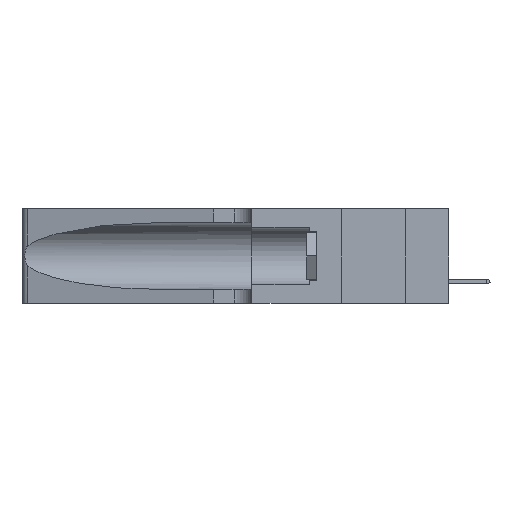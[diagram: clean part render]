
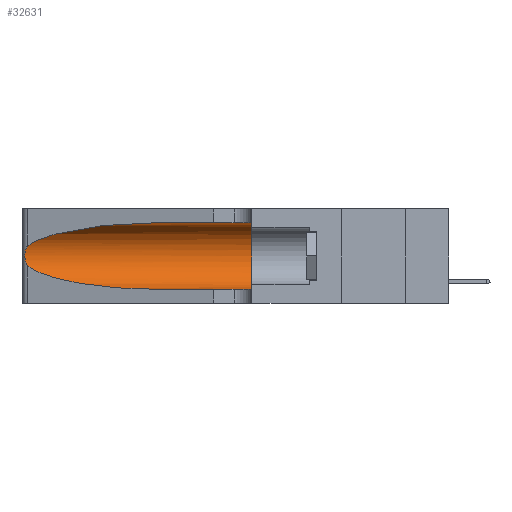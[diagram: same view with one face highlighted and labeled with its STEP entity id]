
A CAD part, left-side view. The second image highlights one B-rep face of the part: STEP entity #32631.
In plain terms, the highlighted cylindrical face has radius 3.308 mm (diameter 6.617 mm), a partial arc.
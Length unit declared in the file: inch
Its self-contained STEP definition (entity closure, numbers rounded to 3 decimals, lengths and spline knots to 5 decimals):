
#422 = CARTESIAN_POINT ( 'NONE',  ( 0.26017, 1.23833, 0.17102 ) ) ;
#545 = EDGE_CURVE ( 'NONE', #37888, #43125, #31810, .T. ) ;
#982 = VERTEX_POINT ( 'NONE', #29966 ) ;
#1101 = CARTESIAN_POINT ( 'NONE',  ( 0.1305, 1.61858, 0.05475 ) ) ;
#1634 = VERTEX_POINT ( 'NONE', #4740 ) ;
#1874 = DIRECTION ( 'NONE',  ( 0., -1., 0. ) ) ;
#2997 = VERTEX_POINT ( 'NONE', #22173 ) ;
#4637 = CARTESIAN_POINT ( 'NONE',  ( 0.25487, 1.22718, 0.22369 ) ) ;
#4740 = CARTESIAN_POINT ( 'NONE',  ( 0.1305, 0.72297, 0.31525 ) ) ;
#6205 = AXIS2_PLACEMENT_3D ( 'NONE', #44078, #36789, #33046 ) ;
#6620 = FACE_OUTER_BOUND ( 'NONE', #32983, .T. ) ;
#6722 = ORIENTED_EDGE ( 'NONE', *, *, #46724, .T. ) ;
#7858 = CARTESIAN_POINT ( 'NONE',  ( 0.25789, 1.23486, 0.15765 ) ) ;
#9179 = CARTESIAN_POINT ( 'NONE',  ( 0.1305, 1.61858, 0.185 ) ) ;
#10398 = EDGE_CURVE ( 'NONE', #982, #2997, #11980, .T. ) ;
#11980 =( BOUNDED_CURVE ( )  B_SPLINE_CURVE ( 3, ( #13541, #35560, #21111, #28175 ),
 .UNSPECIFIED., .F., .F. ) 
 B_SPLINE_CURVE_WITH_KNOTS ( ( 4, 4 ),
 ( 3.44316, 4.71239 ),
 .UNSPECIFIED. ) 
 CURVE ( )  GEOMETRIC_REPRESENTATION_ITEM ( )  RATIONAL_B_SPLINE_CURVE ( ( 1., 0.87, 0.87, 1. ) ) 
 REPRESENTATION_ITEM ( '' )  );
#12842 = ORIENTED_EDGE ( 'NONE', *, *, #17609, .F. ) ;
#13142 = VERTEX_POINT ( 'NONE', #40072 ) ;
#13541 = CARTESIAN_POINT ( 'NONE',  ( 0.25487, 1.22718, 0.14631 ) ) ;
#13623 = ORIENTED_EDGE ( 'NONE', *, *, #23162, .T. ) ;
#14616 = LINE ( 'NONE', #41097, #32411 ) ;
#14864 = LINE ( 'NONE', #1101, #34340 ) ;
#15486 = CARTESIAN_POINT ( 'NONE',  ( 0.25856, 1.23593, 0.16098 ) ) ;
#17253 = AXIS2_PLACEMENT_3D ( 'NONE', #9179, #1874, #26870 ) ;
#17609 = EDGE_CURVE ( 'NONE', #1634, #37888, #14616, .T. ) ;
#18834 = CARTESIAN_POINT ( 'NONE',  ( 0.25555, 1.22993, 0.14849 ) ) ;
#19293 = CARTESIAN_POINT ( 'NONE',  ( 0.2373, 1.15595, 0.28018 ) ) ;
#19314 = CARTESIAN_POINT ( 'NONE',  ( 0.25639, 1.23184, 0.21858 ) ) ;
#19523 = DIRECTION ( 'NONE',  ( 0., -1., 0. ) ) ;
#19613 = CARTESIAN_POINT ( 'NONE',  ( 0.25487, 1.22718, 0.22369 ) ) ;
#20536 = B_SPLINE_CURVE_WITH_KNOTS ( 'NONE', 3,
 ( #4637, #40883, #19314, #30247, #33598, #33901, #44627, #26228, #422, #15486, #7858, #22690, #18834, #41204 ),
 .UNSPECIFIED., .F., .F.,
 ( 4, 2, 2, 2, 2, 2, 4 ),
 ( 0., 0.00027, 0.00053, 0.00107, 0.0016, 0.00187, 0.00214 ),
 .UNSPECIFIED. ) ;
#20895 = EDGE_CURVE ( 'NONE', #2997, #43125, #14864, .T. ) ;
#21111 = CARTESIAN_POINT ( 'NONE',  ( 0.18966, 0.96281, 0.05475 ) ) ;
#21895 = CARTESIAN_POINT ( 'NONE',  ( 0.1305, 0.35, 0.31525 ) ) ;
#22173 = CARTESIAN_POINT ( 'NONE',  ( 0.1305, 0.72297, 0.05475 ) ) ;
#22690 = CARTESIAN_POINT ( 'NONE',  ( 0.25639, 1.23186, 0.15144 ) ) ;
#22770 = ORIENTED_EDGE ( 'NONE', *, *, #545, .F. ) ;
#23162 = EDGE_CURVE ( 'NONE', #1634, #13142, #36978, .T. ) ;
#23308 = CARTESIAN_POINT ( 'NONE',  ( 0.18966, 0.96281, 0.31525 ) ) ;
#23467 = CARTESIAN_POINT ( 'NONE',  ( 0.1305, 0.72297, 0.31525 ) ) ;
#24343 = CYLINDRICAL_SURFACE ( 'NONE', #17253, 0.13025 ) ;
#26228 = CARTESIAN_POINT ( 'NONE',  ( 0.26075, 1.23896, 0.178 ) ) ;
#26870 = DIRECTION ( 'NONE',  ( 0., 0., -1. ) ) ;
#28175 = CARTESIAN_POINT ( 'NONE',  ( 0.1305, 0.72297, 0.05475 ) ) ;
#29966 = CARTESIAN_POINT ( 'NONE',  ( 0.25487, 1.22718, 0.14631 ) ) ;
#30247 = CARTESIAN_POINT ( 'NONE',  ( 0.25787, 1.23484, 0.2124 ) ) ;
#31810 = CIRCLE ( 'NONE', #6205, 0.13025 ) ;
#32411 = VECTOR ( 'NONE', #19523, 39.37008 ) ;
#32631 = ADVANCED_FACE ( 'NONE', ( #6620 ), #24343, .F. ) ;
#32983 = EDGE_LOOP ( 'NONE', ( #13623, #6722, #38938, #36609, #22770, #12842 ) ) ;
#33046 = DIRECTION ( 'NONE',  ( 0., 0., 1. ) ) ;
#33598 = CARTESIAN_POINT ( 'NONE',  ( 0.25854, 1.2359, 0.20912 ) ) ;
#33901 = CARTESIAN_POINT ( 'NONE',  ( 0.26018, 1.23835, 0.19895 ) ) ;
#34340 = VECTOR ( 'NONE', #42458, 39.37008 ) ;
#35560 = CARTESIAN_POINT ( 'NONE',  ( 0.2373, 1.15595, 0.08982 ) ) ;
#36609 = ORIENTED_EDGE ( 'NONE', *, *, #20895, .T. ) ;
#36789 = DIRECTION ( 'NONE',  ( 0., 1., 0. ) ) ;
#36978 =( BOUNDED_CURVE ( )  B_SPLINE_CURVE ( 3, ( #23467, #23308, #19293, #19613 ),
 .UNSPECIFIED., .F., .T. ) 
 B_SPLINE_CURVE_WITH_KNOTS ( ( 4, 4 ),
 ( 1.5708, 2.84003 ),
 .UNSPECIFIED. ) 
 CURVE ( )  GEOMETRIC_REPRESENTATION_ITEM ( )  RATIONAL_B_SPLINE_CURVE ( ( 1., 0.87, 0.87, 1. ) ) 
 REPRESENTATION_ITEM ( '' )  );
#37888 = VERTEX_POINT ( 'NONE', #21895 ) ;
#38938 = ORIENTED_EDGE ( 'NONE', *, *, #10398, .T. ) ;
#40072 = CARTESIAN_POINT ( 'NONE',  ( 0.25487, 1.22718, 0.22369 ) ) ;
#40883 = CARTESIAN_POINT ( 'NONE',  ( 0.25555, 1.22994, 0.2215 ) ) ;
#41097 = CARTESIAN_POINT ( 'NONE',  ( 0.1305, 1.61858, 0.31525 ) ) ;
#41204 = CARTESIAN_POINT ( 'NONE',  ( 0.25487, 1.22718, 0.14631 ) ) ;
#42458 = DIRECTION ( 'NONE',  ( 0., -1., 0. ) ) ;
#43125 = VERTEX_POINT ( 'NONE', #46614 ) ;
#44078 = CARTESIAN_POINT ( 'NONE',  ( 0.1305, 0.35, 0.185 ) ) ;
#44627 = CARTESIAN_POINT ( 'NONE',  ( 0.26075, 1.23896, 0.19203 ) ) ;
#46614 = CARTESIAN_POINT ( 'NONE',  ( 0.1305, 0.35, 0.05475 ) ) ;
#46724 = EDGE_CURVE ( 'NONE', #13142, #982, #20536, .T. ) ;
